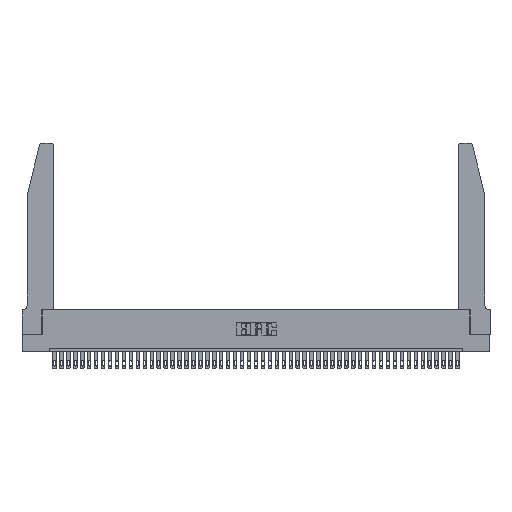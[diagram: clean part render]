
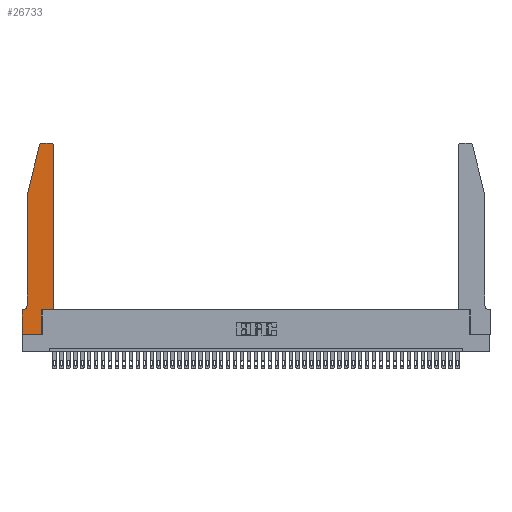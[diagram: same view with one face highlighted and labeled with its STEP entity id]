
A CAD part, top view. The second image highlights one B-rep face of the part: STEP entity #26733.
In plain terms, the highlighted planar face has unit normal (0, 0, 1).
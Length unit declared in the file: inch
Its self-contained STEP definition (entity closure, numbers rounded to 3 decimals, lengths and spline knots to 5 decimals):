
#52 = CARTESIAN_POINT ( 'NONE',  ( 0.4505, 0.35, 0.37 ) ) ;
#1228 = EDGE_CURVE ( 'NONE', #26694, #12107, #24411, .T. ) ;
#1251 = LINE ( 'NONE', #27561, #41943 ) ;
#1415 = CARTESIAN_POINT ( 'NONE',  ( 0.284, 2.75, 0.37 ) ) ;
#2298 = DIRECTION ( 'NONE',  ( 0., -1., 0. ) ) ;
#3039 = EDGE_CURVE ( 'NONE', #26334, #40672, #29933, .T. ) ;
#3294 = EDGE_CURVE ( 'NONE', #12107, #11134, #34971, .T. ) ;
#3395 = EDGE_CURVE ( 'NONE', #11134, #21095, #17463, .T. ) ;
#3464 = CARTESIAN_POINT ( 'NONE',  ( 0.0055, 0.35, 0.37 ) ) ;
#3516 = ORIENTED_EDGE ( 'NONE', *, *, #3395, .T. ) ;
#3657 = DIRECTION ( 'NONE',  ( 1., 0., 0. ) ) ;
#3793 = DIRECTION ( 'NONE',  ( 0., 0., 1. ) ) ;
#5161 = VECTOR ( 'NONE', #9400, 39.37008 ) ;
#5746 = EDGE_CURVE ( 'NONE', #38881, #26694, #36953, .T. ) ;
#5757 = CARTESIAN_POINT ( 'NONE',  ( 0.2865, 0.35, 0.37 ) ) ;
#6091 = CARTESIAN_POINT ( 'NONE',  ( 0.2865, 0.35, 0.37 ) ) ;
#6195 = VECTOR ( 'NONE', #14261, 39.37008 ) ;
#6378 = DIRECTION ( 'NONE',  ( -0.239, -0.971, 0. ) ) ;
#7258 = CARTESIAN_POINT ( 'NONE',  ( 0.2865, 0., 0.37 ) ) ;
#7372 = CARTESIAN_POINT ( 'NONE',  ( 0.0755, 0.35, 0.37 ) ) ;
#7575 = CARTESIAN_POINT ( 'NONE',  ( 0.284, 2.72, 0.37 ) ) ;
#7720 = CARTESIAN_POINT ( 'NONE',  ( 0., 0., 0.37 ) ) ;
#8569 = CARTESIAN_POINT ( 'NONE',  ( 0.0755, 2., 0.37 ) ) ;
#8692 = LINE ( 'NONE', #7372, #38627 ) ;
#9224 = CARTESIAN_POINT ( 'NONE',  ( 0.4205, 2.75, 0.37 ) ) ;
#9373 = ORIENTED_EDGE ( 'NONE', *, *, #5746, .T. ) ;
#9400 = DIRECTION ( 'NONE',  ( -1., 0., 0. ) ) ;
#10595 = VERTEX_POINT ( 'NONE', #41606 ) ;
#10711 = EDGE_CURVE ( 'NONE', #10595, #38881, #1251, .T. ) ;
#11134 = VERTEX_POINT ( 'NONE', #52 ) ;
#11667 = ORIENTED_EDGE ( 'NONE', *, *, #34694, .T. ) ;
#12107 = VERTEX_POINT ( 'NONE', #5757 ) ;
#12136 = FACE_OUTER_BOUND ( 'NONE', #15673, .T. ) ;
#12844 = VECTOR ( 'NONE', #44407, 39.37008 ) ;
#13098 = ORIENTED_EDGE ( 'NONE', *, *, #21978, .T. ) ;
#13649 = VECTOR ( 'NONE', #31348, 39.37008 ) ;
#13984 = LINE ( 'NONE', #8569, #12844 ) ;
#14261 = DIRECTION ( 'NONE',  ( 1., 0., 0. ) ) ;
#15625 = CARTESIAN_POINT ( 'NONE',  ( 0.0755, 0.42, 0.37 ) ) ;
#15673 = EDGE_LOOP ( 'NONE', ( #34688, #13098, #29835, #11667, #16443, #41069, #25975, #9373, #46413, #28585, #3516, #20586 ) ) ;
#16328 = VECTOR ( 'NONE', #29737, 39.37008 ) ;
#16394 = VERTEX_POINT ( 'NONE', #9224 ) ;
#16443 = ORIENTED_EDGE ( 'NONE', *, *, #30366, .T. ) ;
#16495 = CARTESIAN_POINT ( 'NONE',  ( 0.4505, 2.72, 0.37 ) ) ;
#17463 = LINE ( 'NONE', #40465, #16328 ) ;
#17603 = CIRCLE ( 'NONE', #39190, 0.03 ) ;
#17933 = CARTESIAN_POINT ( 'NONE',  ( 0.0055, 0.42, 0.37 ) ) ;
#18136 = LINE ( 'NONE', #46167, #5161 ) ;
#18175 = AXIS2_PLACEMENT_3D ( 'NONE', #27445, #31520, #42254 ) ;
#18299 = DIRECTION ( 'NONE',  ( 1., 0., 0. ) ) ;
#18457 = AXIS2_PLACEMENT_3D ( 'NONE', #36299, #39622, #3657 ) ;
#19799 = EDGE_CURVE ( 'NONE', #21095, #16394, #38274, .T. ) ;
#20586 = ORIENTED_EDGE ( 'NONE', *, *, #19799, .T. ) ;
#21095 = VERTEX_POINT ( 'NONE', #16495 ) ;
#21596 = DIRECTION ( 'NONE',  ( 0., 0., -1. ) ) ;
#21978 = EDGE_CURVE ( 'NONE', #33511, #26334, #17603, .T. ) ;
#24411 = LINE ( 'NONE', #6091, #13649 ) ;
#25975 = ORIENTED_EDGE ( 'NONE', *, *, #10711, .T. ) ;
#26334 = VERTEX_POINT ( 'NONE', #41418 ) ;
#26694 = VERTEX_POINT ( 'NONE', #7258 ) ;
#26733 = ADVANCED_FACE ( 'NONE', ( #12136 ), #29077, .T. ) ;
#27354 = CIRCLE ( 'NONE', #31879, 0.07 ) ;
#27408 = EDGE_CURVE ( 'NONE', #39230, #10595, #8692, .T. ) ;
#27445 = CARTESIAN_POINT ( 'NONE',  ( 0.4205, 2.72, 0.37 ) ) ;
#27561 = CARTESIAN_POINT ( 'NONE',  ( 0., 0., 0.37 ) ) ;
#28033 = CARTESIAN_POINT ( 'NONE',  ( 0.0755, 2., 0.37 ) ) ;
#28585 = ORIENTED_EDGE ( 'NONE', *, *, #3294, .T. ) ;
#28638 = VERTEX_POINT ( 'NONE', #15625 ) ;
#29077 = PLANE ( 'NONE',  #18457 ) ;
#29737 = DIRECTION ( 'NONE',  ( 0., 1., 0. ) ) ;
#29835 = ORIENTED_EDGE ( 'NONE', *, *, #3039, .T. ) ;
#29933 = LINE ( 'NONE', #28033, #45172 ) ;
#30366 = EDGE_CURVE ( 'NONE', #28638, #39230, #27354, .T. ) ;
#31348 = DIRECTION ( 'NONE',  ( 0., 1., 0. ) ) ;
#31520 = DIRECTION ( 'NONE',  ( 0., 0., 1. ) ) ;
#31879 = AXIS2_PLACEMENT_3D ( 'NONE', #17933, #21596, #46827 ) ;
#32601 = EDGE_CURVE ( 'NONE', #16394, #33511, #18136, .T. ) ;
#32826 = DIRECTION ( 'NONE',  ( 1., 0., 0. ) ) ;
#33441 = DIRECTION ( 'NONE',  ( -1., 0., 0. ) ) ;
#33511 = VERTEX_POINT ( 'NONE', #1415 ) ;
#34262 = CARTESIAN_POINT ( 'NONE',  ( 0.0755, 2., 0.37 ) ) ;
#34688 = ORIENTED_EDGE ( 'NONE', *, *, #32601, .T. ) ;
#34694 = EDGE_CURVE ( 'NONE', #40672, #28638, #13984, .T. ) ;
#34971 = LINE ( 'NONE', #35870, #6195 ) ;
#35870 = CARTESIAN_POINT ( 'NONE',  ( 0.4505, 0.35, 0.37 ) ) ;
#36299 = CARTESIAN_POINT ( 'NONE',  ( 0., 0.35, 0.37 ) ) ;
#36399 = VECTOR ( 'NONE', #32826, 39.37008 ) ;
#36637 = CARTESIAN_POINT ( 'NONE',  ( 0., 0., 0.37 ) ) ;
#36953 = LINE ( 'NONE', #7720, #36399 ) ;
#38274 = CIRCLE ( 'NONE', #18175, 0.03 ) ;
#38627 = VECTOR ( 'NONE', #33441, 39.37008 ) ;
#38881 = VERTEX_POINT ( 'NONE', #36637 ) ;
#39190 = AXIS2_PLACEMENT_3D ( 'NONE', #7575, #3793, #18299 ) ;
#39230 = VERTEX_POINT ( 'NONE', #3464 ) ;
#39622 = DIRECTION ( 'NONE',  ( 0., 0., 1. ) ) ;
#40465 = CARTESIAN_POINT ( 'NONE',  ( 0.4505, 0.35, 0.37 ) ) ;
#40672 = VERTEX_POINT ( 'NONE', #34262 ) ;
#41069 = ORIENTED_EDGE ( 'NONE', *, *, #27408, .T. ) ;
#41418 = CARTESIAN_POINT ( 'NONE',  ( 0.25487, 2.72718, 0.37 ) ) ;
#41606 = CARTESIAN_POINT ( 'NONE',  ( 0., 0.35, 0.37 ) ) ;
#41943 = VECTOR ( 'NONE', #2298, 39.37008 ) ;
#42254 = DIRECTION ( 'NONE',  ( 1., 0., 0. ) ) ;
#44407 = DIRECTION ( 'NONE',  ( 0., -1., 0. ) ) ;
#45172 = VECTOR ( 'NONE', #6378, 39.37008 ) ;
#46167 = CARTESIAN_POINT ( 'NONE',  ( 0.2605, 2.75, 0.37 ) ) ;
#46413 = ORIENTED_EDGE ( 'NONE', *, *, #1228, .T. ) ;
#46827 = DIRECTION ( 'NONE',  ( -1., 0., 0. ) ) ;
